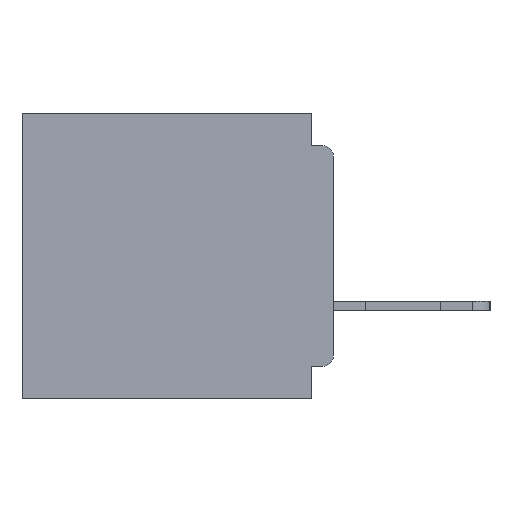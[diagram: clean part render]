
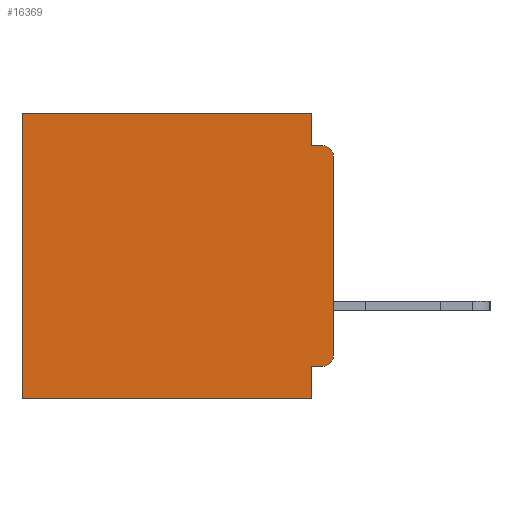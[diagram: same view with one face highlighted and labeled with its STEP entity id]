
A CAD part, left-side view. The second image highlights one B-rep face of the part: STEP entity #16369.
In plain terms, the highlighted planar face has unit normal (-1, 0, 0).
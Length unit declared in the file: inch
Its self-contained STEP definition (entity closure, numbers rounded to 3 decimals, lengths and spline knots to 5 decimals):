
#1019 = DIRECTION ( 'NONE',  ( -1., 0., 0. ) ) ;
#1937 = VECTOR ( 'NONE', #26742, 39.37008 ) ;
#1956 = ORIENTED_EDGE ( 'NONE', *, *, #20438, .T. ) ;
#2118 = VECTOR ( 'NONE', #42046, 39.37008 ) ;
#3189 = DIRECTION ( 'NONE',  ( 0., 0., -1. ) ) ;
#3299 = LINE ( 'NONE', #47136, #11878 ) ;
#4032 = DIRECTION ( 'NONE',  ( 1., 0., 0. ) ) ;
#5314 = VECTOR ( 'NONE', #3189, 39.37008 ) ;
#5996 = LINE ( 'NONE', #32136, #43501 ) ;
#6660 = DIRECTION ( 'NONE',  ( 0., 1., 0. ) ) ;
#7391 = CARTESIAN_POINT ( 'NONE',  ( 0.3, 0.437, -0.4 ) ) ;
#7751 = VERTEX_POINT ( 'NONE', #44310 ) ;
#7764 = ORIENTED_EDGE ( 'NONE', *, *, #19600, .F. ) ;
#8137 = EDGE_CURVE ( 'NONE', #13165, #21869, #29083, .T. ) ;
#9351 = CARTESIAN_POINT ( 'NONE',  ( 0.3, 0.437, -0.4 ) ) ;
#9775 = CARTESIAN_POINT ( 'NONE',  ( 0.3, 0.015, -0.045 ) ) ;
#10624 = CARTESIAN_POINT ( 'NONE',  ( 0.3, 0.015, -0.06 ) ) ;
#10931 = ORIENTED_EDGE ( 'NONE', *, *, #46208, .T. ) ;
#11227 = CARTESIAN_POINT ( 'NONE',  ( 0.3, 0., -0.4 ) ) ;
#11615 = CARTESIAN_POINT ( 'NONE',  ( 0.3, 0., -0.4 ) ) ;
#11843 = LINE ( 'NONE', #9351, #2118 ) ;
#11878 = VECTOR ( 'NONE', #32790, 39.37008 ) ;
#12063 = CARTESIAN_POINT ( 'NONE',  ( 0.3, 0., -0.045 ) ) ;
#13165 = VERTEX_POINT ( 'NONE', #41550 ) ;
#14301 = DIRECTION ( 'NONE',  ( 0., 0., -1. ) ) ;
#14562 = ORIENTED_EDGE ( 'NONE', *, *, #45870, .F. ) ;
#15867 = CARTESIAN_POINT ( 'NONE',  ( 0.3, 0.015, -0.355 ) ) ;
#16369 = ADVANCED_FACE ( 'NONE', ( #24477 ), #25891, .F. ) ;
#17325 = VERTEX_POINT ( 'NONE', #32299 ) ;
#17839 = VECTOR ( 'NONE', #17994, 39.37008 ) ;
#17994 = DIRECTION ( 'NONE',  ( 0., 0., -1. ) ) ;
#18035 = VERTEX_POINT ( 'NONE', #36346 ) ;
#18327 = VERTEX_POINT ( 'NONE', #34449 ) ;
#19102 = ORIENTED_EDGE ( 'NONE', *, *, #38180, .F. ) ;
#19600 = EDGE_CURVE ( 'NONE', #17325, #22378, #34375, .T. ) ;
#20427 = AXIS2_PLACEMENT_3D ( 'NONE', #22925, #1019, #26578 ) ;
#20438 = EDGE_CURVE ( 'NONE', #23334, #23408, #43872, .T. ) ;
#20747 = ORIENTED_EDGE ( 'NONE', *, *, #28477, .F. ) ;
#21869 = VERTEX_POINT ( 'NONE', #7391 ) ;
#21990 = CARTESIAN_POINT ( 'NONE',  ( 0.3, 0., -0.355 ) ) ;
#22378 = VERTEX_POINT ( 'NONE', #28498 ) ;
#22925 = CARTESIAN_POINT ( 'NONE',  ( 0.3, 0.015, -0.34 ) ) ;
#23018 = EDGE_CURVE ( 'NONE', #18035, #46758, #28588, .T. ) ;
#23334 = VERTEX_POINT ( 'NONE', #15867 ) ;
#23408 = VERTEX_POINT ( 'NONE', #31607 ) ;
#24477 = FACE_OUTER_BOUND ( 'NONE', #44447, .T. ) ;
#25048 = CARTESIAN_POINT ( 'NONE',  ( 0.3, 0.031, 0. ) ) ;
#25092 = AXIS2_PLACEMENT_3D ( 'NONE', #10624, #36048, #14301 ) ;
#25626 = DIRECTION ( 'NONE',  ( 0., 1., 0. ) ) ;
#25891 = PLANE ( 'NONE',  #30636 ) ;
#26578 = DIRECTION ( 'NONE',  ( 0., 0., -1. ) ) ;
#26742 = DIRECTION ( 'NONE',  ( 0., -1., 0. ) ) ;
#27527 = LINE ( 'NONE', #36241, #17839 ) ;
#27834 = LINE ( 'NONE', #21990, #45926 ) ;
#28477 = EDGE_CURVE ( 'NONE', #18327, #13165, #3299, .T. ) ;
#28498 = CARTESIAN_POINT ( 'NONE',  ( 0.3, 0.031, -0.045 ) ) ;
#28588 = CIRCLE ( 'NONE', #25092, 0.015 ) ;
#29083 = LINE ( 'NONE', #11615, #39846 ) ;
#29526 = DIRECTION ( 'NONE',  ( 0., 0., -1. ) ) ;
#30636 = AXIS2_PLACEMENT_3D ( 'NONE', #11227, #4032, #29526 ) ;
#30924 = EDGE_CURVE ( 'NONE', #17325, #7751, #5996, .T. ) ;
#31244 = EDGE_CURVE ( 'NONE', #22378, #46758, #39522, .T. ) ;
#31607 = CARTESIAN_POINT ( 'NONE',  ( 0.3, 0., -0.34 ) ) ;
#32136 = CARTESIAN_POINT ( 'NONE',  ( 0.3, 0., 0. ) ) ;
#32299 = CARTESIAN_POINT ( 'NONE',  ( 0.3, 0.031, 0. ) ) ;
#32790 = DIRECTION ( 'NONE',  ( 0., 0., -1. ) ) ;
#33077 = ORIENTED_EDGE ( 'NONE', *, *, #30924, .T. ) ;
#33420 = DIRECTION ( 'NONE',  ( 0., 1., 0. ) ) ;
#34375 = LINE ( 'NONE', #25048, #5314 ) ;
#34449 = CARTESIAN_POINT ( 'NONE',  ( 0.3, 0.031, -0.355 ) ) ;
#35922 = ORIENTED_EDGE ( 'NONE', *, *, #8137, .F. ) ;
#36048 = DIRECTION ( 'NONE',  ( -1., 0., 0. ) ) ;
#36241 = CARTESIAN_POINT ( 'NONE',  ( 0.3, 0., -0.4 ) ) ;
#36346 = CARTESIAN_POINT ( 'NONE',  ( 0.3, 0., -0.06 ) ) ;
#36974 = ORIENTED_EDGE ( 'NONE', *, *, #31244, .F. ) ;
#38180 = EDGE_CURVE ( 'NONE', #18035, #23408, #27527, .T. ) ;
#39522 = LINE ( 'NONE', #12063, #1937 ) ;
#39846 = VECTOR ( 'NONE', #33420, 39.37008 ) ;
#41550 = CARTESIAN_POINT ( 'NONE',  ( 0.3, 0.031, -0.4 ) ) ;
#41785 = ORIENTED_EDGE ( 'NONE', *, *, #23018, .T. ) ;
#42046 = DIRECTION ( 'NONE',  ( 0., 0., -1. ) ) ;
#43501 = VECTOR ( 'NONE', #6660, 39.37008 ) ;
#43872 = CIRCLE ( 'NONE', #20427, 0.015 ) ;
#44310 = CARTESIAN_POINT ( 'NONE',  ( 0.3, 0.437, 0. ) ) ;
#44447 = EDGE_LOOP ( 'NONE', ( #19102, #41785, #36974, #7764, #33077, #10931, #35922, #20747, #14562, #1956 ) ) ;
#45870 = EDGE_CURVE ( 'NONE', #23334, #18327, #27834, .T. ) ;
#45926 = VECTOR ( 'NONE', #25626, 39.37008 ) ;
#46208 = EDGE_CURVE ( 'NONE', #7751, #21869, #11843, .T. ) ;
#46758 = VERTEX_POINT ( 'NONE', #9775 ) ;
#47136 = CARTESIAN_POINT ( 'NONE',  ( 0.3, 0.031, -0.4 ) ) ;
